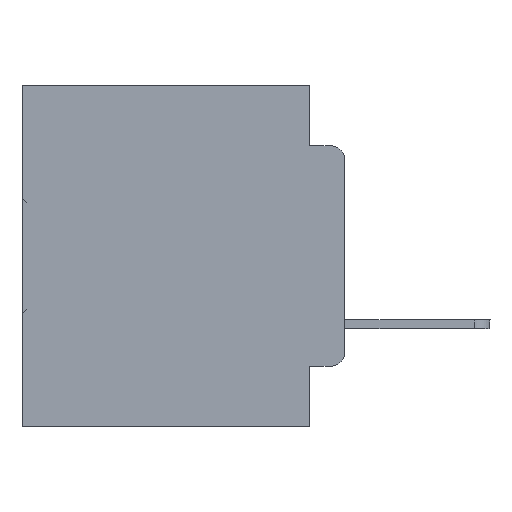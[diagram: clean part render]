
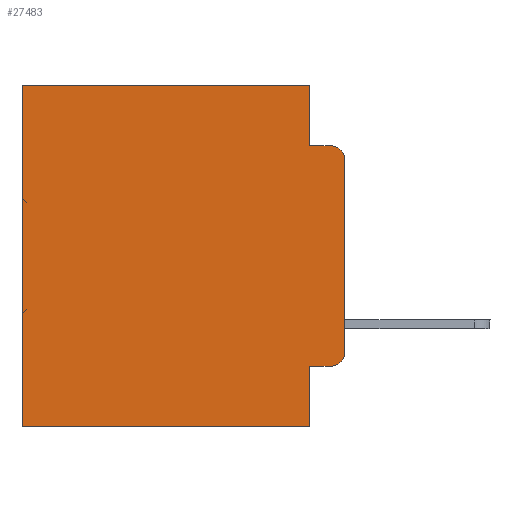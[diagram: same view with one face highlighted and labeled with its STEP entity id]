
A CAD part, left-side view. The second image highlights one B-rep face of the part: STEP entity #27483.
In plain terms, the highlighted planar face has unit normal (-1, 0, 0).
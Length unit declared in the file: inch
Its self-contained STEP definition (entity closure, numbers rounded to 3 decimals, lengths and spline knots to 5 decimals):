
#341 = DIRECTION ( 'NONE',  ( 0., -1., 0. ) ) ;
#1117 = LINE ( 'NONE', #13689, #30506 ) ;
#1365 = CARTESIAN_POINT ( 'NONE',  ( 0.298, 0.051, -0.4115 ) ) ;
#2358 = ORIENTED_EDGE ( 'NONE', *, *, #18250, .T. ) ;
#2469 = CARTESIAN_POINT ( 'NONE',  ( 0.298, 0.051, 0. ) ) ;
#2537 = EDGE_CURVE ( 'NONE', #11780, #31123, #1117, .T. ) ;
#2645 = AXIS2_PLACEMENT_3D ( 'NONE', #3577, #6635, #11777 ) ;
#3577 = CARTESIAN_POINT ( 'NONE',  ( 0.298, 0.02, -0.1085 ) ) ;
#3665 = VECTOR ( 'NONE', #21817, 39.37008 ) ;
#3851 = CARTESIAN_POINT ( 'NONE',  ( 0.298, 0.051, -0.5 ) ) ;
#3932 = DIRECTION ( 'NONE',  ( 0., 1., 0. ) ) ;
#4696 = DIRECTION ( 'NONE',  ( 0., 0., -1. ) ) ;
#4947 = CARTESIAN_POINT ( 'NONE',  ( 0.298, 0.473, 0. ) ) ;
#5294 = DIRECTION ( 'NONE',  ( 0., -1., 0. ) ) ;
#5602 = CARTESIAN_POINT ( 'NONE',  ( 0.298, 0.02, -0.4115 ) ) ;
#6016 = CIRCLE ( 'NONE', #2645, 0.02 ) ;
#6492 = VERTEX_POINT ( 'NONE', #22913 ) ;
#6635 = DIRECTION ( 'NONE',  ( -1., 0., 0. ) ) ;
#6775 = LINE ( 'NONE', #7173, #12506 ) ;
#7173 = CARTESIAN_POINT ( 'NONE',  ( 0.298, 0., 0. ) ) ;
#8123 = VECTOR ( 'NONE', #3932, 39.37008 ) ;
#9149 = CARTESIAN_POINT ( 'NONE',  ( 0.298, 0., -0.5 ) ) ;
#11049 = ORIENTED_EDGE ( 'NONE', *, *, #17211, .F. ) ;
#11220 = DIRECTION ( 'NONE',  ( 0., 0., -1. ) ) ;
#11548 = FACE_OUTER_BOUND ( 'NONE', #12859, .T. ) ;
#11777 = DIRECTION ( 'NONE',  ( 0., 0., -1. ) ) ;
#11780 = VERTEX_POINT ( 'NONE', #2469 ) ;
#12429 = EDGE_CURVE ( 'NONE', #19801, #12915, #18267, .T. ) ;
#12506 = VECTOR ( 'NONE', #30818, 39.37008 ) ;
#12602 = CIRCLE ( 'NONE', #22618, 0.02 ) ;
#12859 = EDGE_LOOP ( 'NONE', ( #11049, #2358, #28672, #18619, #14077, #22483, #14839, #29718, #22980, #31495 ) ) ;
#12915 = VERTEX_POINT ( 'NONE', #5602 ) ;
#13589 = VERTEX_POINT ( 'NONE', #15215 ) ;
#13689 = CARTESIAN_POINT ( 'NONE',  ( 0.298, 0.051, 0. ) ) ;
#14046 = EDGE_CURVE ( 'NONE', #11780, #6492, #33840, .T. ) ;
#14077 = ORIENTED_EDGE ( 'NONE', *, *, #14046, .T. ) ;
#14169 = CARTESIAN_POINT ( 'NONE',  ( 0.298, 0.051, 0. ) ) ;
#14825 = LINE ( 'NONE', #27219, #21025 ) ;
#14839 = ORIENTED_EDGE ( 'NONE', *, *, #24337, .F. ) ;
#15215 = CARTESIAN_POINT ( 'NONE',  ( 0.298, 0.473, -0.5 ) ) ;
#16185 = CARTESIAN_POINT ( 'NONE',  ( 0.298, 0., 0. ) ) ;
#17211 = EDGE_CURVE ( 'NONE', #19089, #17433, #6775, .T. ) ;
#17433 = VERTEX_POINT ( 'NONE', #23209 ) ;
#17470 = DIRECTION ( 'NONE',  ( 0., 1., 0. ) ) ;
#17526 = CARTESIAN_POINT ( 'NONE',  ( 0.298, 0., -0.1085 ) ) ;
#17680 = VERTEX_POINT ( 'NONE', #3851 ) ;
#18250 = EDGE_CURVE ( 'NONE', #19089, #27705, #6016, .T. ) ;
#18267 = LINE ( 'NONE', #18556, #29373 ) ;
#18486 = EDGE_CURVE ( 'NONE', #12915, #17433, #12602, .T. ) ;
#18556 = CARTESIAN_POINT ( 'NONE',  ( 0.298, 0.051, -0.4115 ) ) ;
#18619 = ORIENTED_EDGE ( 'NONE', *, *, #2537, .F. ) ;
#19089 = VERTEX_POINT ( 'NONE', #17526 ) ;
#19226 = AXIS2_PLACEMENT_3D ( 'NONE', #16185, #32468, #11220 ) ;
#19801 = VERTEX_POINT ( 'NONE', #1365 ) ;
#20484 = CARTESIAN_POINT ( 'NONE',  ( 0.298, 0.02, -0.3915 ) ) ;
#20962 = DIRECTION ( 'NONE',  ( 0., 0., -1. ) ) ;
#21025 = VECTOR ( 'NONE', #341, 39.37008 ) ;
#21817 = DIRECTION ( 'NONE',  ( 0., 0., -1. ) ) ;
#22012 = EDGE_CURVE ( 'NONE', #19801, #17680, #26383, .T. ) ;
#22022 = LINE ( 'NONE', #4947, #26942 ) ;
#22483 = ORIENTED_EDGE ( 'NONE', *, *, #31447, .T. ) ;
#22618 = AXIS2_PLACEMENT_3D ( 'NONE', #20484, #25544, #4696 ) ;
#22913 = CARTESIAN_POINT ( 'NONE',  ( 0.298, 0.473, 0. ) ) ;
#22980 = ORIENTED_EDGE ( 'NONE', *, *, #12429, .T. ) ;
#23209 = CARTESIAN_POINT ( 'NONE',  ( 0.298, 0., -0.3915 ) ) ;
#24337 = EDGE_CURVE ( 'NONE', #17680, #13589, #27451, .T. ) ;
#24756 = DIRECTION ( 'NONE',  ( 0., 0., -1. ) ) ;
#25544 = DIRECTION ( 'NONE',  ( -1., 0., 0. ) ) ;
#26383 = LINE ( 'NONE', #14169, #3665 ) ;
#26942 = VECTOR ( 'NONE', #20962, 39.37008 ) ;
#27219 = CARTESIAN_POINT ( 'NONE',  ( 0.298, 0.051, -0.0885 ) ) ;
#27451 = LINE ( 'NONE', #9149, #8123 ) ;
#27483 = ADVANCED_FACE ( 'NONE', ( #11548 ), #29575, .F. ) ;
#27705 = VERTEX_POINT ( 'NONE', #32702 ) ;
#28080 = CARTESIAN_POINT ( 'NONE',  ( 0.298, 0., 0. ) ) ;
#28351 = EDGE_CURVE ( 'NONE', #31123, #27705, #14825, .T. ) ;
#28672 = ORIENTED_EDGE ( 'NONE', *, *, #28351, .F. ) ;
#29154 = CARTESIAN_POINT ( 'NONE',  ( 0.298, 0.051, -0.0885 ) ) ;
#29256 = VECTOR ( 'NONE', #17470, 39.37008 ) ;
#29373 = VECTOR ( 'NONE', #5294, 39.37008 ) ;
#29575 = PLANE ( 'NONE',  #19226 ) ;
#29718 = ORIENTED_EDGE ( 'NONE', *, *, #22012, .F. ) ;
#30506 = VECTOR ( 'NONE', #24756, 39.37008 ) ;
#30818 = DIRECTION ( 'NONE',  ( 0., 0., -1. ) ) ;
#31123 = VERTEX_POINT ( 'NONE', #29154 ) ;
#31447 = EDGE_CURVE ( 'NONE', #6492, #13589, #22022, .T. ) ;
#31495 = ORIENTED_EDGE ( 'NONE', *, *, #18486, .T. ) ;
#32468 = DIRECTION ( 'NONE',  ( 1., 0., 0. ) ) ;
#32702 = CARTESIAN_POINT ( 'NONE',  ( 0.298, 0.02, -0.0885 ) ) ;
#33840 = LINE ( 'NONE', #28080, #29256 ) ;
